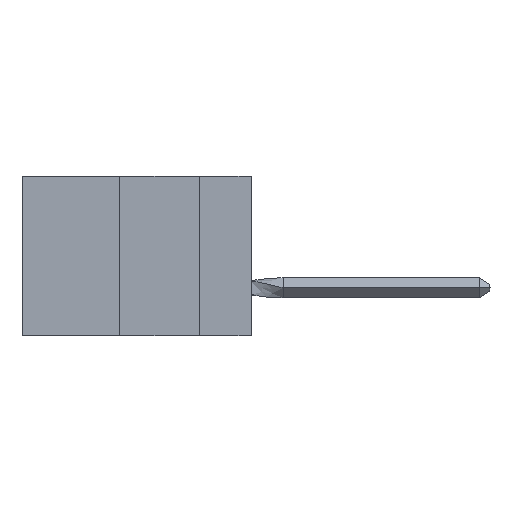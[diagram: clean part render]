
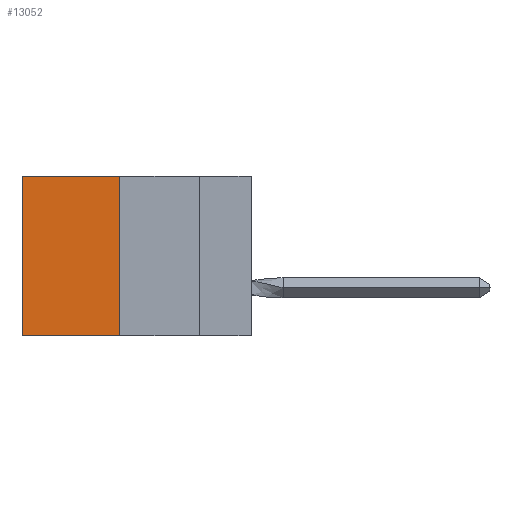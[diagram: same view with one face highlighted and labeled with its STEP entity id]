
A CAD part, left-side view. The second image highlights one B-rep face of the part: STEP entity #13052.
In plain terms, the highlighted planar face has unit normal (-1, 0, 0).
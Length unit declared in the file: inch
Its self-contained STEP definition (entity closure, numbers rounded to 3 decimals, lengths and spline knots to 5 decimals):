
#1211 = EDGE_LOOP ( 'NONE', ( #3399, #18442, #9951, #6660 ) ) ;
#1268 = CARTESIAN_POINT ( 'NONE',  ( 0.305, 0.413, 0. ) ) ;
#1624 = VECTOR ( 'NONE', #18715, 39.37008 ) ;
#1856 = EDGE_CURVE ( 'NONE', #10195, #18008, #7350, .T. ) ;
#1964 = VECTOR ( 'NONE', #6680, 39.37008 ) ;
#3399 = ORIENTED_EDGE ( 'NONE', *, *, #6554, .T. ) ;
#3995 = VECTOR ( 'NONE', #12316, 39.37008 ) ;
#4108 = VERTEX_POINT ( 'NONE', #4829 ) ;
#4829 = CARTESIAN_POINT ( 'NONE',  ( 0.305, 0.413, -0.5 ) ) ;
#5209 = PLANE ( 'NONE',  #18147 ) ;
#6150 = EDGE_CURVE ( 'NONE', #4108, #16340, #12236, .T. ) ;
#6438 = DIRECTION ( 'NONE',  ( 0., 0., -1. ) ) ;
#6490 = DIRECTION ( 'NONE',  ( 1., 0., 0. ) ) ;
#6554 = EDGE_CURVE ( 'NONE', #18008, #16340, #18757, .T. ) ;
#6644 = DIRECTION ( 'NONE',  ( 0., 0., -1. ) ) ;
#6660 = ORIENTED_EDGE ( 'NONE', *, *, #1856, .T. ) ;
#6680 = DIRECTION ( 'NONE',  ( 0., 1., 0. ) ) ;
#7350 = LINE ( 'NONE', #1268, #1624 ) ;
#7781 = FACE_OUTER_BOUND ( 'NONE', #1211, .T. ) ;
#7838 = VECTOR ( 'NONE', #6644, 39.37008 ) ;
#8685 = CARTESIAN_POINT ( 'NONE',  ( 0.305, 0.72, -0.5 ) ) ;
#9593 = CARTESIAN_POINT ( 'NONE',  ( 0.305, 0.413, -0.5 ) ) ;
#9951 = ORIENTED_EDGE ( 'NONE', *, *, #14956, .F. ) ;
#10195 = VERTEX_POINT ( 'NONE', #12345 ) ;
#10782 = CARTESIAN_POINT ( 'NONE',  ( 0.305, 0.413, -0.5 ) ) ;
#12236 = LINE ( 'NONE', #9593, #1964 ) ;
#12316 = DIRECTION ( 'NONE',  ( 0., 0., -1. ) ) ;
#12345 = CARTESIAN_POINT ( 'NONE',  ( 0.305, 0.413, 0. ) ) ;
#13052 = ADVANCED_FACE ( 'NONE', ( #7781 ), #5209, .F. ) ;
#14956 = EDGE_CURVE ( 'NONE', #10195, #4108, #17908, .T. ) ;
#15132 = CARTESIAN_POINT ( 'NONE',  ( 0.305, 0.413, -0.5 ) ) ;
#15357 = CARTESIAN_POINT ( 'NONE',  ( 0.305, 0.72, -0.5 ) ) ;
#16340 = VERTEX_POINT ( 'NONE', #8685 ) ;
#17273 = CARTESIAN_POINT ( 'NONE',  ( 0.305, 0.72, 0. ) ) ;
#17908 = LINE ( 'NONE', #10782, #3995 ) ;
#18008 = VERTEX_POINT ( 'NONE', #17273 ) ;
#18147 = AXIS2_PLACEMENT_3D ( 'NONE', #15132, #6490, #6438 ) ;
#18442 = ORIENTED_EDGE ( 'NONE', *, *, #6150, .F. ) ;
#18715 = DIRECTION ( 'NONE',  ( 0., 1., 0. ) ) ;
#18757 = LINE ( 'NONE', #15357, #7838 ) ;
